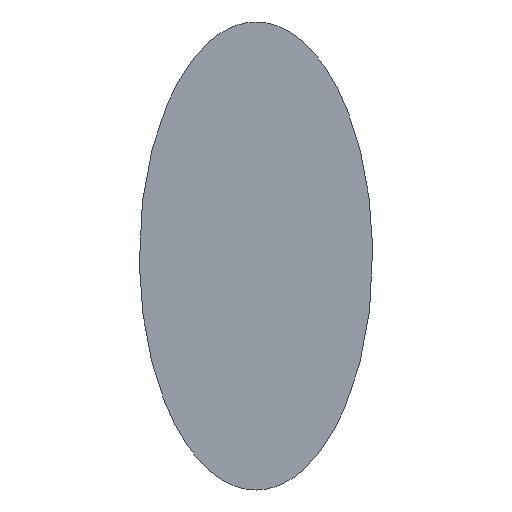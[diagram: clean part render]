
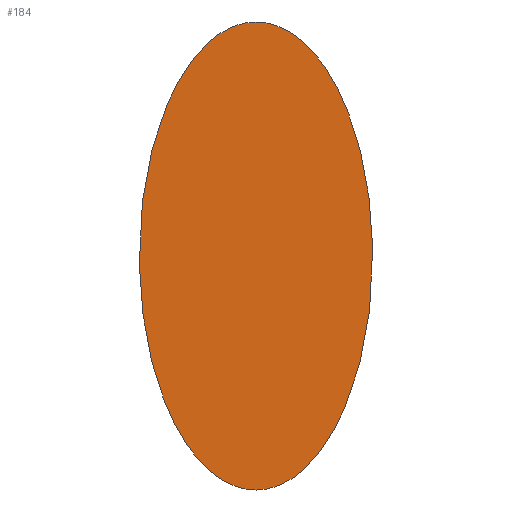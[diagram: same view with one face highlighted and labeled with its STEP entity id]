
A CAD part, front view. The second image highlights one B-rep face of the part: STEP entity #184.
In plain terms, the highlighted planar face has unit normal (0, -1, 0).
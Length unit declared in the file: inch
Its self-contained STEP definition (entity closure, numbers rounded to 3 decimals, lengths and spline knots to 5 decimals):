
#12 = CARTESIAN_POINT ( 'NONE',  ( -0.19765, 0., -0.80356 ) ) ;
#16 = CARTESIAN_POINT ( 'NONE',  ( -0.27206, 0., 0.71083 ) ) ;
#25 = CARTESIAN_POINT ( 'NONE',  ( 0.446, 0., -0.11702 ) ) ;
#34 = ORIENTED_EDGE ( 'NONE', *, *, #362, .F. ) ;
#44 = CARTESIAN_POINT ( 'NONE',  ( 0., 0., -0.894 ) ) ;
#46 = CARTESIAN_POINT ( 'NONE',  ( -0.27206, 0., -0.71083 ) ) ;
#50 = CARTESIAN_POINT ( 'NONE',  ( -0.19765, 0., 0.80356 ) ) ;
#58 = CARTESIAN_POINT ( 'NONE',  ( 0.05838, 0., 0.88824 ) ) ;
#59 = CARTESIAN_POINT ( 'NONE',  ( 0.38971, 0., -0.45024 ) ) ;
#67 = ORIENTED_EDGE ( 'NONE', *, *, #336, .F. ) ;
#75 = CARTESIAN_POINT ( 'NONE',  ( -0.35665, 0., -0.5494 ) ) ;
#79 = CARTESIAN_POINT ( 'NONE',  ( -0.11564, 0., 0.86541 ) ) ;
#86 = CARTESIAN_POINT ( 'NONE',  ( 0.14371, 0., 0.84834 ) ) ;
#87 = CARTESIAN_POINT ( 'NONE',  ( 0.29473, 0., -0.67353 ) ) ;
#104 = CARTESIAN_POINT ( 'NONE',  ( 0., 0., 0. ) ) ;
#107 = CARTESIAN_POINT ( 'NONE',  ( -0.02919, 0., -0.894 ) ) ;
#109 = CARTESIAN_POINT ( 'NONE',  ( -0.43439, 0., -0.234 ) ) ;
#113 = CARTESIAN_POINT ( 'NONE',  ( -0.02919, 0., 0.894 ) ) ;
#118 = CARTESIAN_POINT ( 'NONE',  ( 0.22351, 0., 0.77584 ) ) ;
#120 = CARTESIAN_POINT ( 'NONE',  ( 0.22351, 0., -0.77584 ) ) ;
#140 = CARTESIAN_POINT ( 'NONE',  ( -0.446, 0., 0.11702 ) ) ;
#150 = CARTESIAN_POINT ( 'NONE',  ( 0.29473, 0., 0.67353 ) ) ;
#151 = CARTESIAN_POINT ( 'NONE',  ( 0.14371, 0., -0.84834 ) ) ;
#153 = VERTEX_POINT ( 'NONE', #337 ) ;
#170 = DIRECTION ( 'NONE',  ( 0., 1., 0. ) ) ;
#172 = CARTESIAN_POINT ( 'NONE',  ( 0., 0., -0.894 ) ) ;
#175 = CARTESIAN_POINT ( 'NONE',  ( -0.05838, 0., -0.88824 ) ) ;
#179 = CARTESIAN_POINT ( 'NONE',  ( -0.38971, 0., 0.45024 ) ) ;
#184 = ADVANCED_FACE ( 'NONE', ( #426 ), #295, .F. ) ;
#187 = CARTESIAN_POINT ( 'NONE',  ( 0.38971, 0., 0.45024 ) ) ;
#188 = CARTESIAN_POINT ( 'NONE',  ( 0.05838, 0., -0.88824 ) ) ;
#208 = CARTESIAN_POINT ( 'NONE',  ( -0.14371, 0., -0.84834 ) ) ;
#212 = CARTESIAN_POINT ( 'NONE',  ( -0.29473, 0., 0.67353 ) ) ;
#221 = CARTESIAN_POINT ( 'NONE',  ( 0.446, 0., 0.11702 ) ) ;
#223 = CARTESIAN_POINT ( 'NONE',  ( 0., 0., -0.894 ) ) ;
#241 = CARTESIAN_POINT ( 'NONE',  ( -0.22351, 0., -0.77584 ) ) ;
#245 = CARTESIAN_POINT ( 'NONE',  ( -0.22351, 0., 0.77584 ) ) ;
#252 = EDGE_LOOP ( 'NONE', ( #67, #34 ) ) ;
#254 = CARTESIAN_POINT ( 'NONE',  ( 0.43439, 0., -0.234 ) ) ;
#271 = CARTESIAN_POINT ( 'NONE',  ( -0.29473, 0., -0.67353 ) ) ;
#275 = CARTESIAN_POINT ( 'NONE',  ( -0.14371, 0., 0.84834 ) ) ;
#281 = CARTESIAN_POINT ( 'NONE',  ( 0.11564, 0., 0.86541 ) ) ;
#282 = CARTESIAN_POINT ( 'NONE',  ( 0.35665, 0., -0.5494 ) ) ;
#295 = PLANE ( 'NONE',  #325 ) ;
#302 = CARTESIAN_POINT ( 'NONE',  ( -0.38971, 0., -0.45024 ) ) ;
#308 = CARTESIAN_POINT ( 'NONE',  ( -0.05838, 0., 0.88824 ) ) ;
#314 = VERTEX_POINT ( 'NONE', #172 ) ;
#315 = CARTESIAN_POINT ( 'NONE',  ( 0.19765, 0., 0.80356 ) ) ;
#317 = CARTESIAN_POINT ( 'NONE',  ( 0.27206, 0., -0.71083 ) ) ;
#325 = AXIS2_PLACEMENT_3D ( 'NONE', #104, #170, #405 ) ;
#331 = B_SPLINE_CURVE_WITH_KNOTS ( 'NONE', 3,
 ( #44, #107, #175, #408, #208, #12, #241, #46, #271, #75, #302, #109, #344, #140, #377, #179, #411, #212, #16, #245, #50, #275, #79, #308, #113, #349 ),
 .UNSPECIFIED., .F., .F.,
 ( 4, 2, 2, 2, 2, 2, 2, 2, 2, 2, 2, 2, 4 ),
 ( 0.05519, 0.05863, 0.06206, 0.0655, 0.06894, 0.07581, 0.08268, 0.08955, 0.09642, 0.09986, 0.10329, 0.10673, 0.11017 ),
 .UNSPECIFIED. ) ;
#336 = EDGE_CURVE ( 'NONE', #314, #153, #331, .T. ) ;
#337 = CARTESIAN_POINT ( 'NONE',  ( 0., 0., 0.894 ) ) ;
#344 = CARTESIAN_POINT ( 'NONE',  ( -0.446, 0., -0.11702 ) ) ;
#349 = CARTESIAN_POINT ( 'NONE',  ( 0., 0., 0.894 ) ) ;
#355 = CARTESIAN_POINT ( 'NONE',  ( 0.27206, 0., 0.71083 ) ) ;
#356 = CARTESIAN_POINT ( 'NONE',  ( 0.19765, 0., -0.80356 ) ) ;
#362 = EDGE_CURVE ( 'NONE', #153, #314, #365, .T. ) ;
#365 = B_SPLINE_CURVE_WITH_KNOTS ( 'NONE', 3,
 ( #384, #420, #58, #281, #86, #315, #118, #355, #150, #385, #187, #421, #221, #25, #254, #59, #282, #87, #317, #120, #356, #151, #386, #188, #422, #223 ),
 .UNSPECIFIED., .F., .F.,
 ( 4, 2, 2, 2, 2, 2, 2, 2, 2, 2, 2, 2, 4 ),
 ( 0., 0.00345, 0.0069, 0.01035, 0.0138, 0.0207, 0.0276, 0.0345, 0.04139, 0.04484, 0.04829, 0.05174, 0.05519 ),
 .UNSPECIFIED. ) ;
#377 = CARTESIAN_POINT ( 'NONE',  ( -0.43439, 0., 0.234 ) ) ;
#384 = CARTESIAN_POINT ( 'NONE',  ( 0., 0., 0.894 ) ) ;
#385 = CARTESIAN_POINT ( 'NONE',  ( 0.35665, 0., 0.5494 ) ) ;
#386 = CARTESIAN_POINT ( 'NONE',  ( 0.11564, 0., -0.86541 ) ) ;
#405 = DIRECTION ( 'NONE',  ( 0., 0., 1. ) ) ;
#408 = CARTESIAN_POINT ( 'NONE',  ( -0.11564, 0., -0.86541 ) ) ;
#411 = CARTESIAN_POINT ( 'NONE',  ( -0.35665, 0., 0.5494 ) ) ;
#420 = CARTESIAN_POINT ( 'NONE',  ( 0.02919, 0., 0.894 ) ) ;
#421 = CARTESIAN_POINT ( 'NONE',  ( 0.43439, 0., 0.234 ) ) ;
#422 = CARTESIAN_POINT ( 'NONE',  ( 0.02919, 0., -0.894 ) ) ;
#426 = FACE_OUTER_BOUND ( 'NONE', #252, .T. ) ;
